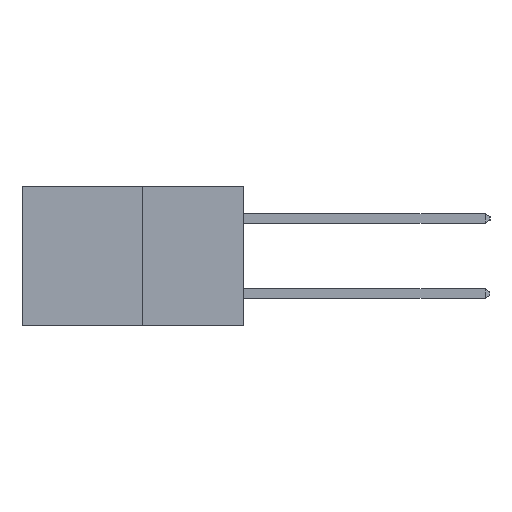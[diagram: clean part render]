
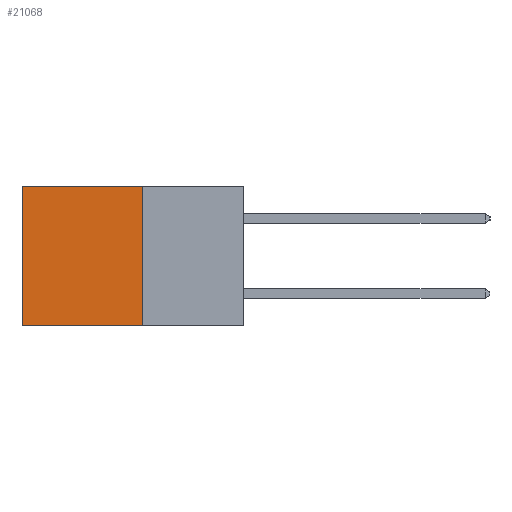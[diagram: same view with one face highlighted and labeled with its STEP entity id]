
A CAD part, left-side view. The second image highlights one B-rep face of the part: STEP entity #21068.
In plain terms, the highlighted planar face has unit normal (-1, 0, 0).
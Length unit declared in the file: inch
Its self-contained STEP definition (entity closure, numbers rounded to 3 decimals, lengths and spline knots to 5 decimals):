
#853 = CARTESIAN_POINT ( 'NONE',  ( 0.277, 0.27, -0.37 ) ) ;
#2764 = ORIENTED_EDGE ( 'NONE', *, *, #14539, .F. ) ;
#2918 = PLANE ( 'NONE',  #6670 ) ;
#4836 = CARTESIAN_POINT ( 'NONE',  ( 0.277, 0.27, 0. ) ) ;
#4923 = DIRECTION ( 'NONE',  ( 1., 0., 0. ) ) ;
#5132 = EDGE_CURVE ( 'NONE', #21295, #5245, #5835, .T. ) ;
#5245 = VERTEX_POINT ( 'NONE', #14981 ) ;
#5418 = VECTOR ( 'NONE', #16274, 39.37008 ) ;
#5835 = LINE ( 'NONE', #24431, #6453 ) ;
#6420 = CARTESIAN_POINT ( 'NONE',  ( 0.277, 0.59, -0.37 ) ) ;
#6453 = VECTOR ( 'NONE', #12733, 39.37008 ) ;
#6670 = AXIS2_PLACEMENT_3D ( 'NONE', #853, #4923, #18737 ) ;
#6958 = CARTESIAN_POINT ( 'NONE',  ( 0.277, 0.27, -0.37 ) ) ;
#7056 = DIRECTION ( 'NONE',  ( 0., 0., -1. ) ) ;
#7192 = ORIENTED_EDGE ( 'NONE', *, *, #5132, .T. ) ;
#8638 = VERTEX_POINT ( 'NONE', #20654 ) ;
#8960 = DIRECTION ( 'NONE',  ( 0., 1., 0. ) ) ;
#9487 = EDGE_LOOP ( 'NONE', ( #21115, #18459, #2764, #7192 ) ) ;
#10577 = VERTEX_POINT ( 'NONE', #14664 ) ;
#10843 = VECTOR ( 'NONE', #8960, 39.37008 ) ;
#10965 = VECTOR ( 'NONE', #7056, 39.37008 ) ;
#12543 = EDGE_CURVE ( 'NONE', #8638, #10577, #21291, .T. ) ;
#12733 = DIRECTION ( 'NONE',  ( 0., 1., 0. ) ) ;
#14539 = EDGE_CURVE ( 'NONE', #21295, #8638, #16857, .T. ) ;
#14664 = CARTESIAN_POINT ( 'NONE',  ( 0.277, 0.59, -0.37 ) ) ;
#14981 = CARTESIAN_POINT ( 'NONE',  ( 0.277, 0.59, 0. ) ) ;
#16274 = DIRECTION ( 'NONE',  ( 0., 0., -1. ) ) ;
#16857 = LINE ( 'NONE', #20810, #10965 ) ;
#17179 = FACE_OUTER_BOUND ( 'NONE', #9487, .T. ) ;
#18459 = ORIENTED_EDGE ( 'NONE', *, *, #12543, .F. ) ;
#18737 = DIRECTION ( 'NONE',  ( 0., 0., -1. ) ) ;
#20654 = CARTESIAN_POINT ( 'NONE',  ( 0.277, 0.27, -0.37 ) ) ;
#20810 = CARTESIAN_POINT ( 'NONE',  ( 0.277, 0.27, -0.37 ) ) ;
#21068 = ADVANCED_FACE ( 'NONE', ( #17179 ), #2918, .F. ) ;
#21115 = ORIENTED_EDGE ( 'NONE', *, *, #21130, .T. ) ;
#21119 = LINE ( 'NONE', #6420, #5418 ) ;
#21130 = EDGE_CURVE ( 'NONE', #5245, #10577, #21119, .T. ) ;
#21291 = LINE ( 'NONE', #6958, #10843 ) ;
#21295 = VERTEX_POINT ( 'NONE', #4836 ) ;
#24431 = CARTESIAN_POINT ( 'NONE',  ( 0.277, 0.27, 0. ) ) ;
